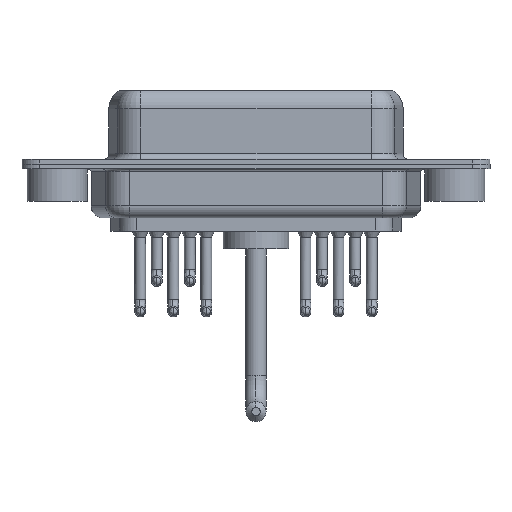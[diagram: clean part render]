
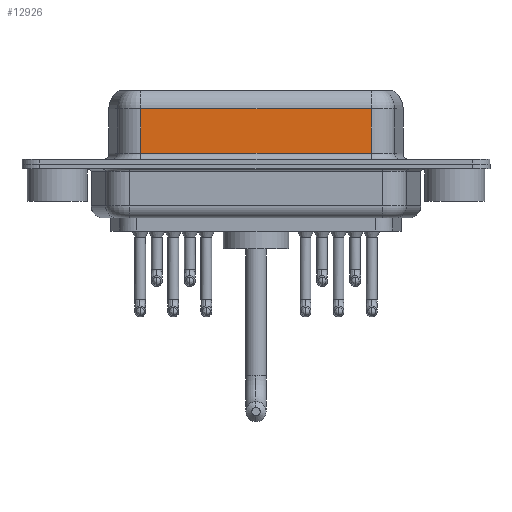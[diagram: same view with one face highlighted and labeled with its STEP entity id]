
A CAD part, front view. The second image highlights one B-rep face of the part: STEP entity #12926.
In plain terms, the highlighted planar face has unit normal (0, -1, 0).
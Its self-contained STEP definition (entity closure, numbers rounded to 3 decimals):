
#518 = VECTOR ( 'NONE', #2017, 1000. ) ;
#1797 = VERTEX_POINT ( 'NONE', #12146 ) ;
#1805 = EDGE_CURVE ( 'NONE', #11514, #14052, #16585, .T. ) ;
#2017 = DIRECTION ( 'NONE',  ( 0., 0., -1. ) ) ;
#2170 = VECTOR ( 'NONE', #5659, 1000. ) ;
#2218 = VERTEX_POINT ( 'NONE', #4558 ) ;
#2355 = ORIENTED_EDGE ( 'NONE', *, *, #2617, .T. ) ;
#2617 = EDGE_CURVE ( 'NONE', #14052, #2218, #6044, .T. ) ;
#3304 = ORIENTED_EDGE ( 'NONE', *, *, #9559, .F. ) ;
#3324 = CARTESIAN_POINT ( 'NONE',  ( 26.287, -3.95, 4.65 ) ) ;
#4558 = CARTESIAN_POINT ( 'NONE',  ( 7.013, -3.95, 0.9 ) ) ;
#5659 = DIRECTION ( 'NONE',  ( 0., 0., -1. ) ) ;
#6044 = LINE ( 'NONE', #7089, #2170 ) ;
#6082 = CARTESIAN_POINT ( 'NONE',  ( 26.287, -3.95, 6.4 ) ) ;
#7089 = CARTESIAN_POINT ( 'NONE',  ( 7.013, -3.95, 6.4 ) ) ;
#8081 = EDGE_LOOP ( 'NONE', ( #3304, #11723, #2355, #18688 ) ) ;
#8102 = CARTESIAN_POINT ( 'NONE',  ( 7.013, -3.95, 4.65 ) ) ;
#8499 = VECTOR ( 'NONE', #13386, 1000. ) ;
#8663 = EDGE_CURVE ( 'NONE', #2218, #1797, #15736, .T. ) ;
#9508 = CARTESIAN_POINT ( 'NONE',  ( 26.287, -3.95, 6.4 ) ) ;
#9559 = EDGE_CURVE ( 'NONE', #11514, #1797, #15006, .T. ) ;
#9958 = DIRECTION ( 'NONE',  ( 1., 0., 0. ) ) ;
#10390 = CARTESIAN_POINT ( 'NONE',  ( 26.287, -3.95, 4.65 ) ) ;
#10933 = PLANE ( 'NONE',  #15429 ) ;
#11514 = VERTEX_POINT ( 'NONE', #10390 ) ;
#11723 = ORIENTED_EDGE ( 'NONE', *, *, #1805, .T. ) ;
#12146 = CARTESIAN_POINT ( 'NONE',  ( 26.287, -3.95, 0.9 ) ) ;
#12449 = DIRECTION ( 'NONE',  ( 0., 1., 0. ) ) ;
#12926 = ADVANCED_FACE ( 'NONE', ( #18124 ), #10933, .F. ) ;
#13386 = DIRECTION ( 'NONE',  ( -1., 0., 0. ) ) ;
#14052 = VERTEX_POINT ( 'NONE', #8102 ) ;
#15006 = LINE ( 'NONE', #6082, #518 ) ;
#15429 = AXIS2_PLACEMENT_3D ( 'NONE', #9508, #12449, #18210 ) ;
#15736 = LINE ( 'NONE', #17050, #18002 ) ;
#16585 = LINE ( 'NONE', #3324, #8499 ) ;
#17050 = CARTESIAN_POINT ( 'NONE',  ( 26.287, -3.95, 0.9 ) ) ;
#18002 = VECTOR ( 'NONE', #9958, 1000. ) ;
#18124 = FACE_OUTER_BOUND ( 'NONE', #8081, .T. ) ;
#18210 = DIRECTION ( 'NONE',  ( 0., 0., 1. ) ) ;
#18688 = ORIENTED_EDGE ( 'NONE', *, *, #8663, .T. ) ;
